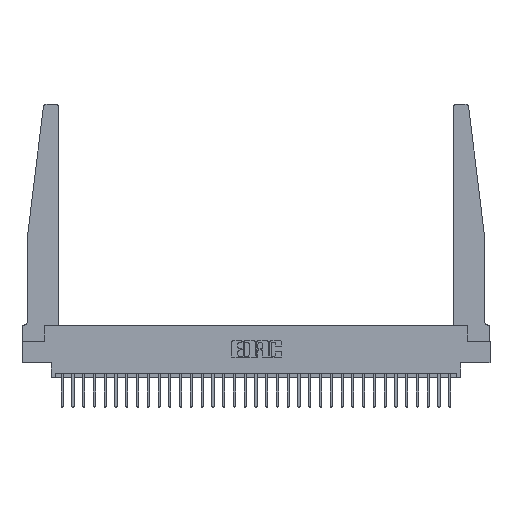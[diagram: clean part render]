
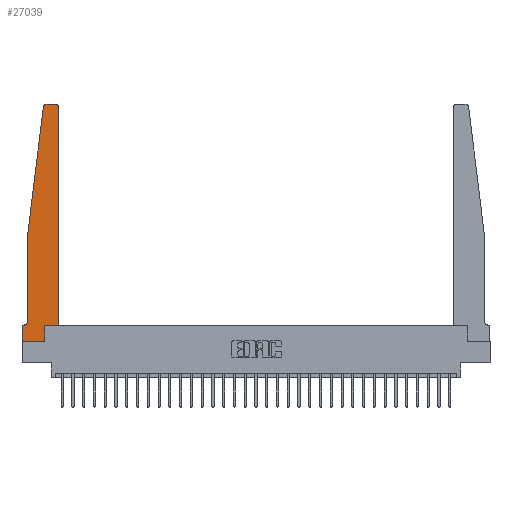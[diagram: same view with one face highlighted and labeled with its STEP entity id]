
A CAD part, top view. The second image highlights one B-rep face of the part: STEP entity #27039.
In plain terms, the highlighted planar face has unit normal (0, 0, 1).
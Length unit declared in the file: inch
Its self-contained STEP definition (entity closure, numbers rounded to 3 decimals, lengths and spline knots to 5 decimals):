
#378 = CARTESIAN_POINT ( 'NONE',  ( 0.425, 2.72, 0.37 ) ) ;
#449 = LINE ( 'NONE', #24191, #18045 ) ;
#1272 = EDGE_CURVE ( 'NONE', #19855, #2199, #12876, .T. ) ;
#1505 = VECTOR ( 'NONE', #11283, 39.37008 ) ;
#1569 = DIRECTION ( 'NONE',  ( 0., -1., 0. ) ) ;
#1740 = EDGE_LOOP ( 'NONE', ( #25688, #20662, #22063, #17450, #16724, #26197, #27851, #20795, #9659, #19625, #9499, #28824 ) ) ;
#1819 = EDGE_CURVE ( 'NONE', #16122, #8734, #22130, .T. ) ;
#2199 = VERTEX_POINT ( 'NONE', #2696 ) ;
#2418 = DIRECTION ( 'NONE',  ( 0., 0., -1. ) ) ;
#2696 = CARTESIAN_POINT ( 'NONE',  ( 0.2605, 0.18, 0.37 ) ) ;
#2697 = VERTEX_POINT ( 'NONE', #13456 ) ;
#2803 = VERTEX_POINT ( 'NONE', #13940 ) ;
#2939 = PLANE ( 'NONE',  #13272 ) ;
#3828 = VECTOR ( 'NONE', #19868, 39.37008 ) ;
#3955 = LINE ( 'NONE', #4939, #16147 ) ;
#4444 = VERTEX_POINT ( 'NONE', #24472 ) ;
#4939 = CARTESIAN_POINT ( 'NONE',  ( 0.065, 0.1875, 0.37 ) ) ;
#5283 = DIRECTION ( 'NONE',  ( 0., 0., 1. ) ) ;
#5913 = EDGE_CURVE ( 'NONE', #13604, #2697, #3955, .T. ) ;
#6070 = DIRECTION ( 'NONE',  ( 0., 0., 1. ) ) ;
#6304 = AXIS2_PLACEMENT_3D ( 'NONE', #22429, #8697, #24745 ) ;
#6488 = VECTOR ( 'NONE', #1569, 39.37008 ) ;
#7208 = CARTESIAN_POINT ( 'NONE',  ( 0.015, 0.1875, 0.37 ) ) ;
#8134 = DIRECTION ( 'NONE',  ( 0., -1., 0. ) ) ;
#8389 = DIRECTION ( 'NONE',  ( 0., 1., 0. ) ) ;
#8453 = LINE ( 'NONE', #11630, #20656 ) ;
#8613 = VERTEX_POINT ( 'NONE', #26089 ) ;
#8697 = DIRECTION ( 'NONE',  ( 0., 0., 1. ) ) ;
#8734 = VERTEX_POINT ( 'NONE', #10529 ) ;
#8909 = VECTOR ( 'NONE', #12498, 39.37008 ) ;
#8950 = CARTESIAN_POINT ( 'NONE',  ( 0.065, 1.25, 0.37 ) ) ;
#9034 = EDGE_CURVE ( 'NONE', #2803, #13030, #8453, .T. ) ;
#9499 = ORIENTED_EDGE ( 'NONE', *, *, #9034, .T. ) ;
#9659 = ORIENTED_EDGE ( 'NONE', *, *, #1272, .T. ) ;
#9677 = CARTESIAN_POINT ( 'NONE',  ( 0.24675, 2.72367, 0.37 ) ) ;
#10529 = CARTESIAN_POINT ( 'NONE',  ( 0.27653, 2.75, 0.37 ) ) ;
#10823 = LINE ( 'NONE', #26832, #21559 ) ;
#10922 = EDGE_CURVE ( 'NONE', #29214, #12490, #19793, .T. ) ;
#11283 = DIRECTION ( 'NONE',  ( -0.122, -0.992, 0. ) ) ;
#11630 = CARTESIAN_POINT ( 'NONE',  ( 0.425, 0.18, 0.37 ) ) ;
#12490 = VERTEX_POINT ( 'NONE', #23797 ) ;
#12498 = DIRECTION ( 'NONE',  ( 1., 0., 0. ) ) ;
#12592 = CARTESIAN_POINT ( 'NONE',  ( 0.25, 2.75, 0.37 ) ) ;
#12761 = CARTESIAN_POINT ( 'NONE',  ( 0.395, 2.75, 0.37 ) ) ;
#12876 = LINE ( 'NONE', #19789, #24350 ) ;
#13030 = VERTEX_POINT ( 'NONE', #378 ) ;
#13272 = AXIS2_PLACEMENT_3D ( 'NONE', #18987, #5283, #21318 ) ;
#13456 = CARTESIAN_POINT ( 'NONE',  ( 0., 0.1875, 0.37 ) ) ;
#13604 = VERTEX_POINT ( 'NONE', #7208 ) ;
#13808 = EDGE_CURVE ( 'NONE', #2199, #2803, #20365, .T. ) ;
#13915 = DIRECTION ( 'NONE',  ( 0., 1., 0. ) ) ;
#13940 = CARTESIAN_POINT ( 'NONE',  ( 0.425, 0.18, 0.37 ) ) ;
#16114 = EDGE_CURVE ( 'NONE', #12490, #8613, #449, .T. ) ;
#16122 = VERTEX_POINT ( 'NONE', #12761 ) ;
#16147 = VECTOR ( 'NONE', #23283, 39.37008 ) ;
#16169 = CARTESIAN_POINT ( 'NONE',  ( 0.015, 0.2375, 0.37 ) ) ;
#16724 = ORIENTED_EDGE ( 'NONE', *, *, #29613, .T. ) ;
#17426 = EDGE_CURVE ( 'NONE', #4444, #19855, #10823, .T. ) ;
#17440 = FACE_OUTER_BOUND ( 'NONE', #1740, .T. ) ;
#17450 = ORIENTED_EDGE ( 'NONE', *, *, #16114, .T. ) ;
#17558 = DIRECTION ( 'NONE',  ( 1., 0., 0. ) ) ;
#18045 = VECTOR ( 'NONE', #8134, 39.37008 ) ;
#18471 = DIRECTION ( 'NONE',  ( -1., 0., 0. ) ) ;
#18987 = CARTESIAN_POINT ( 'NONE',  ( 0., 0.1875, 0.37 ) ) ;
#19625 = ORIENTED_EDGE ( 'NONE', *, *, #13808, .T. ) ;
#19645 = CARTESIAN_POINT ( 'NONE',  ( 0.2605, 0., 0.37 ) ) ;
#19761 = CARTESIAN_POINT ( 'NONE',  ( 0.395, 2.72, 0.37 ) ) ;
#19789 = CARTESIAN_POINT ( 'NONE',  ( 0.2605, 0.18, 0.37 ) ) ;
#19793 = LINE ( 'NONE', #8950, #1505 ) ;
#19855 = VERTEX_POINT ( 'NONE', #19645 ) ;
#19868 = DIRECTION ( 'NONE',  ( -1., 0., 0. ) ) ;
#20365 = LINE ( 'NONE', #28456, #8909 ) ;
#20656 = VECTOR ( 'NONE', #13915, 39.37008 ) ;
#20662 = ORIENTED_EDGE ( 'NONE', *, *, #22768, .T. ) ;
#20795 = ORIENTED_EDGE ( 'NONE', *, *, #17426, .T. ) ;
#21318 = DIRECTION ( 'NONE',  ( 1., 0., 0. ) ) ;
#21559 = VECTOR ( 'NONE', #17558, 39.37008 ) ;
#22063 = ORIENTED_EDGE ( 'NONE', *, *, #10922, .T. ) ;
#22085 = DIRECTION ( 'NONE',  ( 1., 0., 0. ) ) ;
#22130 = LINE ( 'NONE', #12592, #3828 ) ;
#22429 = CARTESIAN_POINT ( 'NONE',  ( 0.27653, 2.72, 0.37 ) ) ;
#22768 = EDGE_CURVE ( 'NONE', #8734, #29214, #27377, .T. ) ;
#23283 = DIRECTION ( 'NONE',  ( -1., 0., 0. ) ) ;
#23372 = EDGE_CURVE ( 'NONE', #13030, #16122, #24454, .T. ) ;
#23797 = CARTESIAN_POINT ( 'NONE',  ( 0.065, 1.25, 0.37 ) ) ;
#23985 = CIRCLE ( 'NONE', #29281, 0.05 ) ;
#24175 = AXIS2_PLACEMENT_3D ( 'NONE', #19761, #6070, #22085 ) ;
#24191 = CARTESIAN_POINT ( 'NONE',  ( 0.065, 1.25, 0.37 ) ) ;
#24350 = VECTOR ( 'NONE', #8389, 39.37008 ) ;
#24454 = CIRCLE ( 'NONE', #24175, 0.03 ) ;
#24472 = CARTESIAN_POINT ( 'NONE',  ( 0., 0., 0.37 ) ) ;
#24739 = EDGE_CURVE ( 'NONE', #2697, #4444, #24776, .T. ) ;
#24745 = DIRECTION ( 'NONE',  ( 1., 0., 0. ) ) ;
#24776 = LINE ( 'NONE', #29099, #6488 ) ;
#25688 = ORIENTED_EDGE ( 'NONE', *, *, #1819, .T. ) ;
#26089 = CARTESIAN_POINT ( 'NONE',  ( 0.065, 0.2375, 0.37 ) ) ;
#26197 = ORIENTED_EDGE ( 'NONE', *, *, #5913, .T. ) ;
#26832 = CARTESIAN_POINT ( 'NONE',  ( 0., 0., 0.37 ) ) ;
#27039 = ADVANCED_FACE ( 'NONE', ( #17440 ), #2939, .T. ) ;
#27377 = CIRCLE ( 'NONE', #6304, 0.03 ) ;
#27851 = ORIENTED_EDGE ( 'NONE', *, *, #24739, .T. ) ;
#28456 = CARTESIAN_POINT ( 'NONE',  ( 0.425, 0.18, 0.37 ) ) ;
#28824 = ORIENTED_EDGE ( 'NONE', *, *, #23372, .T. ) ;
#29099 = CARTESIAN_POINT ( 'NONE',  ( 0., 0., 0.37 ) ) ;
#29214 = VERTEX_POINT ( 'NONE', #9677 ) ;
#29281 = AXIS2_PLACEMENT_3D ( 'NONE', #16169, #2418, #18471 ) ;
#29613 = EDGE_CURVE ( 'NONE', #8613, #13604, #23985, .T. ) ;
